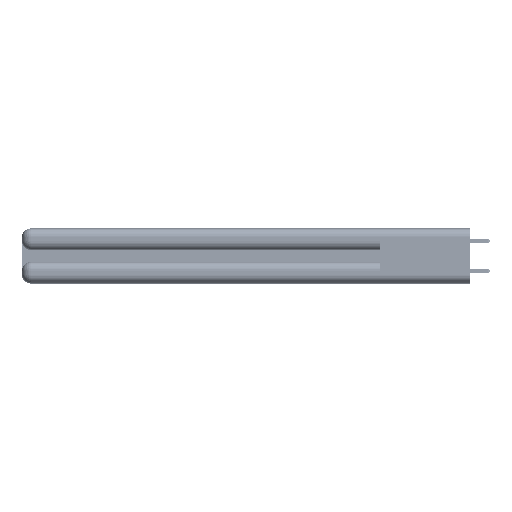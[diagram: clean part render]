
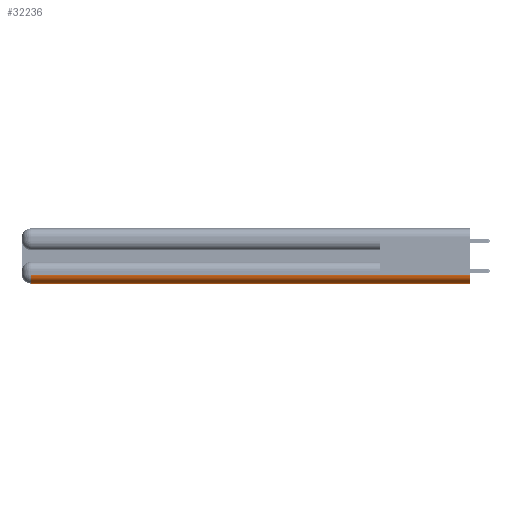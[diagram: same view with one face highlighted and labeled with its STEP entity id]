
A CAD part, left-side view. The second image highlights one B-rep face of the part: STEP entity #32236.
In plain terms, the highlighted cylindrical face has radius 1.524 mm (diameter 3.048 mm), a partial arc.
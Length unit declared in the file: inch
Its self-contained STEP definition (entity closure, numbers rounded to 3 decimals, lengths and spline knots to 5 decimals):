
#241 = CARTESIAN_POINT ( 'NONE',  ( 0.06, 2.94, 0.06 ) ) ;
#2331 = ORIENTED_EDGE ( 'NONE', *, *, #45374, .F. ) ;
#6385 = DIRECTION ( 'NONE',  ( 0., 1., 0. ) ) ;
#8008 = EDGE_CURVE ( 'NONE', #31434, #46779, #52430, .T. ) ;
#8060 = LINE ( 'NONE', #42959, #21593 ) ;
#8665 = ORIENTED_EDGE ( 'NONE', *, *, #34931, .F. ) ;
#9865 = VECTOR ( 'NONE', #16217, 39.37008 ) ;
#10219 = DIRECTION ( 'NONE',  ( 0., -1., 0. ) ) ;
#11144 = AXIS2_PLACEMENT_3D ( 'NONE', #19742, #44242, #20431 ) ;
#13380 = CARTESIAN_POINT ( 'NONE',  ( 0., 2.94, 0.06 ) ) ;
#13475 = AXIS2_PLACEMENT_3D ( 'NONE', #34961, #10219, #51244 ) ;
#15516 = VERTEX_POINT ( 'NONE', #13380 ) ;
#15825 = CARTESIAN_POINT ( 'NONE',  ( 0.06, 0., 0. ) ) ;
#16217 = DIRECTION ( 'NONE',  ( 0., -1., 0. ) ) ;
#17315 = DIRECTION ( 'NONE',  ( 0., 0., 1. ) ) ;
#17403 = EDGE_LOOP ( 'NONE', ( #27226, #8665, #2331, #50667 ) ) ;
#19742 = CARTESIAN_POINT ( 'NONE',  ( 0.06, 0., 0.06 ) ) ;
#20431 = DIRECTION ( 'NONE',  ( 0., 0., 1. ) ) ;
#21060 = DIRECTION ( 'NONE',  ( 0., 1., 0. ) ) ;
#21593 = VECTOR ( 'NONE', #6385, 39.37008 ) ;
#26856 = CYLINDRICAL_SURFACE ( 'NONE', #11144, 0.06 ) ;
#27226 = ORIENTED_EDGE ( 'NONE', *, *, #8008, .F. ) ;
#28038 = AXIS2_PLACEMENT_3D ( 'NONE', #241, #21060, #17315 ) ;
#29411 = FACE_OUTER_BOUND ( 'NONE', #17403, .T. ) ;
#31434 = VERTEX_POINT ( 'NONE', #43633 ) ;
#31489 = CARTESIAN_POINT ( 'NONE',  ( 0.06, 2.94, 0. ) ) ;
#32236 = ADVANCED_FACE ( 'NONE', ( #29411 ), #26856, .T. ) ;
#33257 = EDGE_CURVE ( 'NONE', #46779, #33337, #8060, .T. ) ;
#33337 = VERTEX_POINT ( 'NONE', #31489 ) ;
#34931 = EDGE_CURVE ( 'NONE', #15516, #31434, #49599, .T. ) ;
#34961 = CARTESIAN_POINT ( 'NONE',  ( 0.06, 0., 0.06 ) ) ;
#41104 = CARTESIAN_POINT ( 'NONE',  ( 0., 0., 0.06 ) ) ;
#42959 = CARTESIAN_POINT ( 'NONE',  ( 0.06, 3., 0. ) ) ;
#43633 = CARTESIAN_POINT ( 'NONE',  ( 0., 0., 0.06 ) ) ;
#44242 = DIRECTION ( 'NONE',  ( 0., 1., 0. ) ) ;
#45374 = EDGE_CURVE ( 'NONE', #33337, #15516, #49213, .T. ) ;
#46779 = VERTEX_POINT ( 'NONE', #15825 ) ;
#49213 = CIRCLE ( 'NONE', #28038, 0.06 ) ;
#49599 = LINE ( 'NONE', #41104, #9865 ) ;
#50667 = ORIENTED_EDGE ( 'NONE', *, *, #33257, .F. ) ;
#51244 = DIRECTION ( 'NONE',  ( 0., 0., 1. ) ) ;
#52430 = CIRCLE ( 'NONE', #13475, 0.06 ) ;
